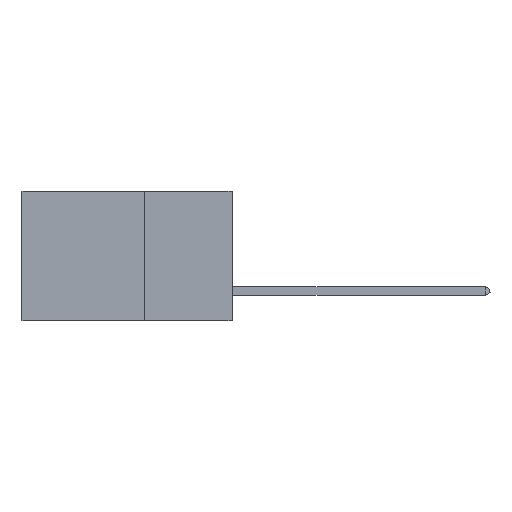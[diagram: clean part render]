
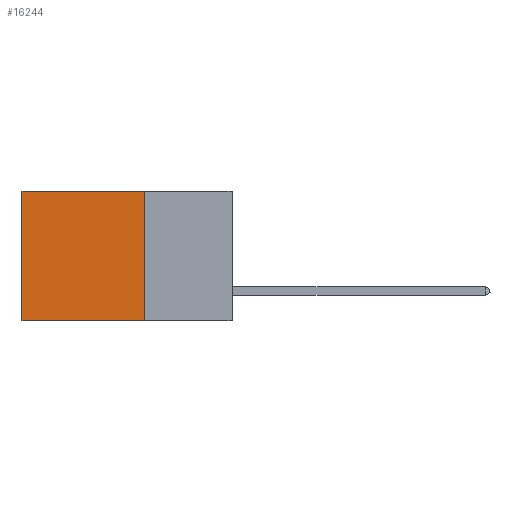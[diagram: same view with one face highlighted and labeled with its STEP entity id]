
A CAD part, left-side view. The second image highlights one B-rep face of the part: STEP entity #16244.
In plain terms, the highlighted planar face has unit normal (-1, 0, 0).
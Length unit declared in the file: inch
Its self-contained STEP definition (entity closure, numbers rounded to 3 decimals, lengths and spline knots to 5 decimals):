
#163 = ORIENTED_EDGE ( 'NONE', *, *, #16048, .T. ) ;
#641 = EDGE_LOOP ( 'NONE', ( #163, #41795, #30329, #27165 ) ) ;
#1192 = CARTESIAN_POINT ( 'NONE',  ( 0.2875, 0.6, -0.37 ) ) ;
#4076 = VERTEX_POINT ( 'NONE', #1192 ) ;
#6805 = VECTOR ( 'NONE', #7599, 39.37008 ) ;
#7599 = DIRECTION ( 'NONE',  ( 0., 0., -1. ) ) ;
#7994 = VERTEX_POINT ( 'NONE', #15693 ) ;
#8713 = VERTEX_POINT ( 'NONE', #14127 ) ;
#9255 = DIRECTION ( 'NONE',  ( 1., 0., 0. ) ) ;
#10325 = LINE ( 'NONE', #36799, #17087 ) ;
#10364 = AXIS2_PLACEMENT_3D ( 'NONE', #12895, #9255, #13033 ) ;
#10654 = CARTESIAN_POINT ( 'NONE',  ( 0.2875, 0.6, 0. ) ) ;
#12443 = DIRECTION ( 'NONE',  ( 0., 1., 0. ) ) ;
#12509 = LINE ( 'NONE', #10654, #6805 ) ;
#12895 = CARTESIAN_POINT ( 'NONE',  ( 0.2875, 0.25, 0. ) ) ;
#13033 = DIRECTION ( 'NONE',  ( 0., 0., -1. ) ) ;
#14127 = CARTESIAN_POINT ( 'NONE',  ( 0.2875, 0.6, 0. ) ) ;
#14240 = VERTEX_POINT ( 'NONE', #15399 ) ;
#14249 = EDGE_CURVE ( 'NONE', #7994, #14240, #32307, .T. ) ;
#15399 = CARTESIAN_POINT ( 'NONE',  ( 0.2875, 0.25, -0.37 ) ) ;
#15642 = FACE_OUTER_BOUND ( 'NONE', #641, .T. ) ;
#15690 = CARTESIAN_POINT ( 'NONE',  ( 0.2875, 0.25, 0. ) ) ;
#15693 = CARTESIAN_POINT ( 'NONE',  ( 0.2875, 0.25, 0. ) ) ;
#16048 = EDGE_CURVE ( 'NONE', #8713, #4076, #12509, .T. ) ;
#16244 = ADVANCED_FACE ( 'NONE', ( #15642 ), #35897, .F. ) ;
#17087 = VECTOR ( 'NONE', #29846, 39.37008 ) ;
#18857 = VECTOR ( 'NONE', #28689, 39.37008 ) ;
#19099 = LINE ( 'NONE', #32119, #28927 ) ;
#27165 = ORIENTED_EDGE ( 'NONE', *, *, #34205, .T. ) ;
#28689 = DIRECTION ( 'NONE',  ( 0., 0., -1. ) ) ;
#28927 = VECTOR ( 'NONE', #12443, 39.37008 ) ;
#29846 = DIRECTION ( 'NONE',  ( 0., 1., 0. ) ) ;
#30329 = ORIENTED_EDGE ( 'NONE', *, *, #14249, .F. ) ;
#32119 = CARTESIAN_POINT ( 'NONE',  ( 0.2875, 0.25, -0.37 ) ) ;
#32307 = LINE ( 'NONE', #15690, #18857 ) ;
#34205 = EDGE_CURVE ( 'NONE', #7994, #8713, #10325, .T. ) ;
#35897 = PLANE ( 'NONE',  #10364 ) ;
#36799 = CARTESIAN_POINT ( 'NONE',  ( 0.2875, 0.25, 0. ) ) ;
#41634 = EDGE_CURVE ( 'NONE', #14240, #4076, #19099, .T. ) ;
#41795 = ORIENTED_EDGE ( 'NONE', *, *, #41634, .F. ) ;
